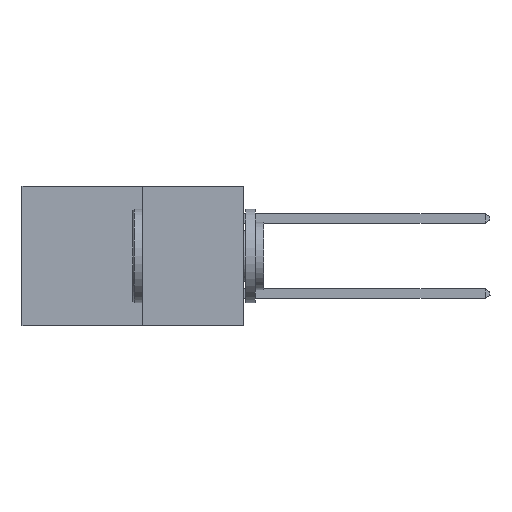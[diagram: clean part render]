
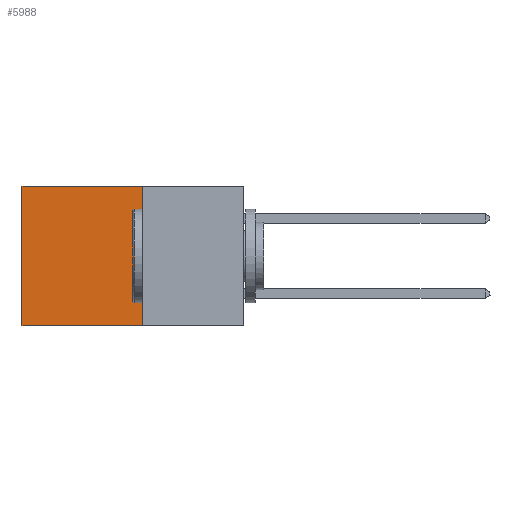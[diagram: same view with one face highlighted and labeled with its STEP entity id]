
A CAD part, left-side view. The second image highlights one B-rep face of the part: STEP entity #5988.
In plain terms, the highlighted planar face has unit normal (-1, 0, 0).
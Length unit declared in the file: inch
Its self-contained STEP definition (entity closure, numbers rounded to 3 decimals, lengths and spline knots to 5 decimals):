
#575 = VERTEX_POINT ( 'NONE', #4616 ) ;
#582 = ORIENTED_EDGE ( 'NONE', *, *, #5931, .F. ) ;
#701 = VECTOR ( 'NONE', #3000, 39.37008 ) ;
#1223 = LINE ( 'NONE', #2375, #1453 ) ;
#1453 = VECTOR ( 'NONE', #8074, 39.37008 ) ;
#1742 = VERTEX_POINT ( 'NONE', #3578 ) ;
#1961 = CARTESIAN_POINT ( 'NONE',  ( 0.277, 0.27, 0. ) ) ;
#2144 = FACE_OUTER_BOUND ( 'NONE', #7735, .T. ) ;
#2269 = ORIENTED_EDGE ( 'NONE', *, *, #9060, .F. ) ;
#2362 = CARTESIAN_POINT ( 'NONE',  ( 0.277, 0.27, -0.37 ) ) ;
#2375 = CARTESIAN_POINT ( 'NONE',  ( 0.277, 0.59, -0.37 ) ) ;
#2587 = LINE ( 'NONE', #5083, #701 ) ;
#2994 = DIRECTION ( 'NONE',  ( 0., 0., -1. ) ) ;
#3000 = DIRECTION ( 'NONE',  ( 0., 1., 0. ) ) ;
#3063 = DIRECTION ( 'NONE',  ( 1., 0., 0. ) ) ;
#3135 = EDGE_CURVE ( 'NONE', #7358, #6181, #1223, .T. ) ;
#3450 = ORIENTED_EDGE ( 'NONE', *, *, #4366, .T. ) ;
#3578 = CARTESIAN_POINT ( 'NONE',  ( 0.277, 0.27, 0. ) ) ;
#3623 = LINE ( 'NONE', #5077, #5257 ) ;
#3882 = CARTESIAN_POINT ( 'NONE',  ( 0.277, 0.59, 0. ) ) ;
#4366 = EDGE_CURVE ( 'NONE', #1742, #7358, #7641, .T. ) ;
#4616 = CARTESIAN_POINT ( 'NONE',  ( 0.277, 0.27, -0.37 ) ) ;
#5077 = CARTESIAN_POINT ( 'NONE',  ( 0.277, 0.27, -0.37 ) ) ;
#5083 = CARTESIAN_POINT ( 'NONE',  ( 0.277, 0.27, -0.37 ) ) ;
#5257 = VECTOR ( 'NONE', #2994, 39.37008 ) ;
#5528 = CARTESIAN_POINT ( 'NONE',  ( 0.277, 0.59, -0.37 ) ) ;
#5798 = VECTOR ( 'NONE', #6183, 39.37008 ) ;
#5931 = EDGE_CURVE ( 'NONE', #575, #6181, #2587, .T. ) ;
#5988 = ADVANCED_FACE ( 'NONE', ( #2144 ), #6518, .F. ) ;
#6181 = VERTEX_POINT ( 'NONE', #5528 ) ;
#6183 = DIRECTION ( 'NONE',  ( 0., 1., 0. ) ) ;
#6322 = ORIENTED_EDGE ( 'NONE', *, *, #3135, .T. ) ;
#6518 = PLANE ( 'NONE',  #7125 ) ;
#7125 = AXIS2_PLACEMENT_3D ( 'NONE', #2362, #3063, #7938 ) ;
#7358 = VERTEX_POINT ( 'NONE', #3882 ) ;
#7641 = LINE ( 'NONE', #1961, #5798 ) ;
#7735 = EDGE_LOOP ( 'NONE', ( #6322, #582, #2269, #3450 ) ) ;
#7938 = DIRECTION ( 'NONE',  ( 0., 0., -1. ) ) ;
#8074 = DIRECTION ( 'NONE',  ( 0., 0., -1. ) ) ;
#9060 = EDGE_CURVE ( 'NONE', #1742, #575, #3623, .T. ) ;
